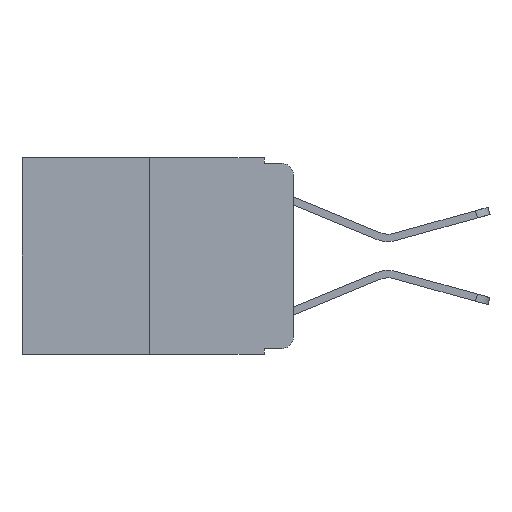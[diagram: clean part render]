
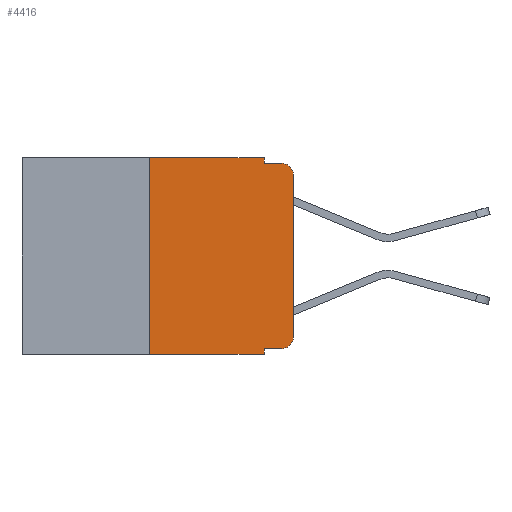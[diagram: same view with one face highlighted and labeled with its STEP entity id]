
A CAD part, left-side view. The second image highlights one B-rep face of the part: STEP entity #4416.
In plain terms, the highlighted planar face has unit normal (-1, 0, 0).
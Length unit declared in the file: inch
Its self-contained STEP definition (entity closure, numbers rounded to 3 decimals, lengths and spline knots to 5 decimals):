
#380 = DIRECTION ( 'NONE',  ( 0., 0., -1. ) ) ;
#597 = AXIS2_PLACEMENT_3D ( 'NONE', #11821, #6149, #380 ) ;
#825 = VECTOR ( 'NONE', #7043, 39.37008 ) ;
#826 = DIRECTION ( 'NONE',  ( 0., 0., -1. ) ) ;
#930 = DIRECTION ( 'NONE',  ( 0., -1., 0. ) ) ;
#1133 = CARTESIAN_POINT ( 'NONE',  ( 0., 0.25, 0. ) ) ;
#1137 = CARTESIAN_POINT ( 'NONE',  ( 0., 0.473, -0.343 ) ) ;
#1426 = ORIENTED_EDGE ( 'NONE', *, *, #4606, .F. ) ;
#1511 = CARTESIAN_POINT ( 'NONE',  ( 0., 0.051, -0.333 ) ) ;
#1588 = AXIS2_PLACEMENT_3D ( 'NONE', #4446, #11134, #5417 ) ;
#1637 = CARTESIAN_POINT ( 'NONE',  ( 0., 0.051, 0. ) ) ;
#1946 = EDGE_CURVE ( 'NONE', #5872, #4718, #5408, .T. ) ;
#2030 = VERTEX_POINT ( 'NONE', #9183 ) ;
#2469 = ORIENTED_EDGE ( 'NONE', *, *, #5371, .F. ) ;
#2512 = LINE ( 'NONE', #7098, #7602 ) ;
#2877 = VECTOR ( 'NONE', #4251, 39.37008 ) ;
#3134 = VERTEX_POINT ( 'NONE', #1637 ) ;
#3251 = EDGE_LOOP ( 'NONE', ( #9216, #9507, #7243, #2469, #10102, #5609, #10984, #1426, #9067, #9372 ) ) ;
#3404 = VERTEX_POINT ( 'NONE', #5854 ) ;
#3429 = CARTESIAN_POINT ( 'NONE',  ( 0., 0.25, 0. ) ) ;
#3625 = CARTESIAN_POINT ( 'NONE',  ( 0., 0.02, -0.333 ) ) ;
#3633 = EDGE_CURVE ( 'NONE', #6782, #5903, #8106, .T. ) ;
#3675 = CARTESIAN_POINT ( 'NONE',  ( 0., 0.473, 0. ) ) ;
#3694 = LINE ( 'NONE', #10710, #6252 ) ;
#3846 = EDGE_CURVE ( 'NONE', #4218, #3134, #9871, .T. ) ;
#3968 = LINE ( 'NONE', #8042, #825 ) ;
#3973 = CARTESIAN_POINT ( 'NONE',  ( 0., 0.051, -0.01 ) ) ;
#4218 = VERTEX_POINT ( 'NONE', #3429 ) ;
#4251 = DIRECTION ( 'NONE',  ( 0., -1., 0. ) ) ;
#4416 = ADVANCED_FACE ( 'NONE', ( #5826 ), #5619, .F. ) ;
#4446 = CARTESIAN_POINT ( 'NONE',  ( 0., 0.02, -0.313 ) ) ;
#4606 = EDGE_CURVE ( 'NONE', #3404, #2030, #3694, .T. ) ;
#4718 = VERTEX_POINT ( 'NONE', #5102 ) ;
#4738 = EDGE_CURVE ( 'NONE', #11400, #4718, #8233, .T. ) ;
#4769 = VECTOR ( 'NONE', #930, 39.37008 ) ;
#4975 = VECTOR ( 'NONE', #6896, 39.37008 ) ;
#4979 = DIRECTION ( 'NONE',  ( 0., 0., -1. ) ) ;
#5102 = CARTESIAN_POINT ( 'NONE',  ( 0., 0.02, -0.01 ) ) ;
#5371 = EDGE_CURVE ( 'NONE', #3134, #5872, #3968, .T. ) ;
#5408 = LINE ( 'NONE', #9056, #2877 ) ;
#5417 = DIRECTION ( 'NONE',  ( 0., 0., -1. ) ) ;
#5609 = ORIENTED_EDGE ( 'NONE', *, *, #8370, .F. ) ;
#5619 = PLANE ( 'NONE',  #11329 ) ;
#5826 = FACE_OUTER_BOUND ( 'NONE', #3251, .T. ) ;
#5845 = VERTEX_POINT ( 'NONE', #8792 ) ;
#5854 = CARTESIAN_POINT ( 'NONE',  ( 0., 0.051, -0.333 ) ) ;
#5872 = VERTEX_POINT ( 'NONE', #3973 ) ;
#5903 = VERTEX_POINT ( 'NONE', #8867 ) ;
#6149 = DIRECTION ( 'NONE',  ( -1., 0., 0. ) ) ;
#6252 = VECTOR ( 'NONE', #4979, 39.37008 ) ;
#6566 = DIRECTION ( 'NONE',  ( 1., 0., 0. ) ) ;
#6674 = CARTESIAN_POINT ( 'NONE',  ( 0., 0.473, 0. ) ) ;
#6782 = VERTEX_POINT ( 'NONE', #3625 ) ;
#6896 = DIRECTION ( 'NONE',  ( 0., 0., 1. ) ) ;
#7043 = DIRECTION ( 'NONE',  ( 0., 0., -1. ) ) ;
#7098 = CARTESIAN_POINT ( 'NONE',  ( 0., 0., 0. ) ) ;
#7243 = ORIENTED_EDGE ( 'NONE', *, *, #1946, .F. ) ;
#7255 = EDGE_CURVE ( 'NONE', #3404, #6782, #9369, .T. ) ;
#7602 = VECTOR ( 'NONE', #9952, 39.37008 ) ;
#8042 = CARTESIAN_POINT ( 'NONE',  ( 0., 0.051, 0. ) ) ;
#8106 = CIRCLE ( 'NONE', #1588, 0.02 ) ;
#8219 = DIRECTION ( 'NONE',  ( 0., -1., 0. ) ) ;
#8233 = CIRCLE ( 'NONE', #597, 0.02 ) ;
#8370 = EDGE_CURVE ( 'NONE', #5845, #4218, #10373, .T. ) ;
#8792 = CARTESIAN_POINT ( 'NONE',  ( 0., 0.25, -0.343 ) ) ;
#8856 = VECTOR ( 'NONE', #10719, 39.37008 ) ;
#8867 = CARTESIAN_POINT ( 'NONE',  ( 0., 0., -0.313 ) ) ;
#9056 = CARTESIAN_POINT ( 'NONE',  ( 0., 0.051, -0.01 ) ) ;
#9067 = ORIENTED_EDGE ( 'NONE', *, *, #7255, .T. ) ;
#9183 = CARTESIAN_POINT ( 'NONE',  ( 0., 0.051, -0.343 ) ) ;
#9216 = ORIENTED_EDGE ( 'NONE', *, *, #12180, .T. ) ;
#9369 = LINE ( 'NONE', #1511, #12134 ) ;
#9370 = CARTESIAN_POINT ( 'NONE',  ( 0., 0., -0.03 ) ) ;
#9372 = ORIENTED_EDGE ( 'NONE', *, *, #3633, .T. ) ;
#9507 = ORIENTED_EDGE ( 'NONE', *, *, #4738, .T. ) ;
#9845 = EDGE_CURVE ( 'NONE', #5845, #2030, #11060, .T. ) ;
#9871 = LINE ( 'NONE', #6674, #4769 ) ;
#9952 = DIRECTION ( 'NONE',  ( 0., 0., 1. ) ) ;
#10102 = ORIENTED_EDGE ( 'NONE', *, *, #3846, .F. ) ;
#10373 = LINE ( 'NONE', #1133, #4975 ) ;
#10710 = CARTESIAN_POINT ( 'NONE',  ( 0., 0.051, 0. ) ) ;
#10719 = DIRECTION ( 'NONE',  ( 0., -1., 0. ) ) ;
#10984 = ORIENTED_EDGE ( 'NONE', *, *, #9845, .T. ) ;
#11060 = LINE ( 'NONE', #1137, #8856 ) ;
#11134 = DIRECTION ( 'NONE',  ( -1., 0., 0. ) ) ;
#11329 = AXIS2_PLACEMENT_3D ( 'NONE', #3675, #6566, #826 ) ;
#11400 = VERTEX_POINT ( 'NONE', #9370 ) ;
#11821 = CARTESIAN_POINT ( 'NONE',  ( 0., 0.02, -0.03 ) ) ;
#12134 = VECTOR ( 'NONE', #8219, 39.37008 ) ;
#12180 = EDGE_CURVE ( 'NONE', #5903, #11400, #2512, .T. ) ;
